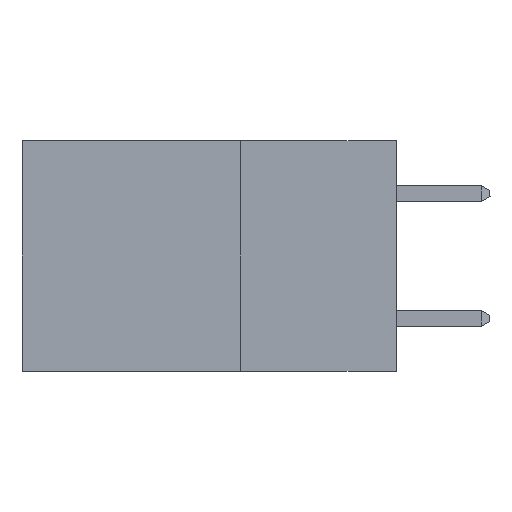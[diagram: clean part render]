
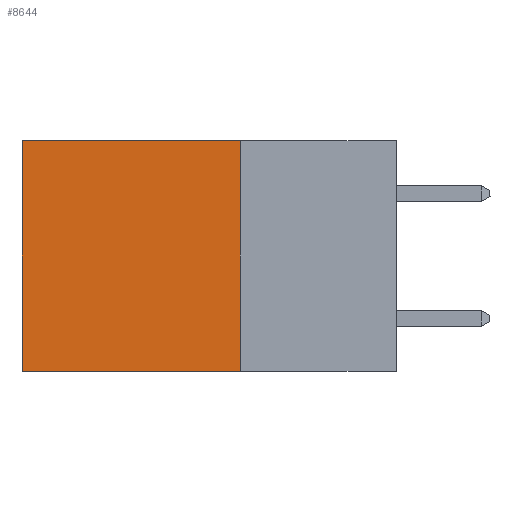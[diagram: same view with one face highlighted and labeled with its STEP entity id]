
A CAD part, left-side view. The second image highlights one B-rep face of the part: STEP entity #8644.
In plain terms, the highlighted planar face has unit normal (-1, 0, 0).
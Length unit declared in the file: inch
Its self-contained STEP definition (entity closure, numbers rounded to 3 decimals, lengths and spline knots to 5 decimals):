
#35 = VECTOR ( 'NONE', #12548, 39.37008 ) ;
#37 = AXIS2_PLACEMENT_3D ( 'NONE', #1441, #10226, #12680 ) ;
#749 = CARTESIAN_POINT ( 'NONE',  ( 0.298, 0.25, 0. ) ) ;
#1441 = CARTESIAN_POINT ( 'NONE',  ( 0.298, 0.25, 0. ) ) ;
#2020 = CARTESIAN_POINT ( 'NONE',  ( 0.298, 0.25, 0. ) ) ;
#2573 = ORIENTED_EDGE ( 'NONE', *, *, #11608, .T. ) ;
#3134 = LINE ( 'NONE', #9184, #35 ) ;
#3535 = EDGE_CURVE ( 'NONE', #3935, #13254, #6602, .T. ) ;
#3663 = DIRECTION ( 'NONE',  ( 0., 0., -1. ) ) ;
#3904 = VERTEX_POINT ( 'NONE', #749 ) ;
#3935 = VERTEX_POINT ( 'NONE', #10319 ) ;
#4289 = LINE ( 'NONE', #2020, #9448 ) ;
#5802 = CARTESIAN_POINT ( 'NONE',  ( 0.298, 0.25, -0.37 ) ) ;
#6526 = EDGE_CURVE ( 'NONE', #7617, #13254, #8835, .T. ) ;
#6602 = LINE ( 'NONE', #11719, #9190 ) ;
#6907 = ORIENTED_EDGE ( 'NONE', *, *, #9926, .F. ) ;
#7183 = ORIENTED_EDGE ( 'NONE', *, *, #6526, .F. ) ;
#7617 = VERTEX_POINT ( 'NONE', #5802 ) ;
#8644 = ADVANCED_FACE ( 'NONE', ( #12233 ), #11887, .F. ) ;
#8835 = LINE ( 'NONE', #12252, #14677 ) ;
#9184 = CARTESIAN_POINT ( 'NONE',  ( 0.298, 0.25, 0. ) ) ;
#9190 = VECTOR ( 'NONE', #3663, 39.37008 ) ;
#9373 = DIRECTION ( 'NONE',  ( 0., 0., -1. ) ) ;
#9448 = VECTOR ( 'NONE', #9373, 39.37008 ) ;
#9926 = EDGE_CURVE ( 'NONE', #3904, #7617, #4289, .T. ) ;
#10226 = DIRECTION ( 'NONE',  ( 1., 0., 0. ) ) ;
#10319 = CARTESIAN_POINT ( 'NONE',  ( 0.298, 0.6, 0. ) ) ;
#11464 = EDGE_LOOP ( 'NONE', ( #13954, #7183, #6907, #2573 ) ) ;
#11608 = EDGE_CURVE ( 'NONE', #3904, #3935, #3134, .T. ) ;
#11719 = CARTESIAN_POINT ( 'NONE',  ( 0.298, 0.6, 0. ) ) ;
#11887 = PLANE ( 'NONE',  #37 ) ;
#12233 = FACE_OUTER_BOUND ( 'NONE', #11464, .T. ) ;
#12252 = CARTESIAN_POINT ( 'NONE',  ( 0.298, 0.25, -0.37 ) ) ;
#12303 = DIRECTION ( 'NONE',  ( 0., 1., 0. ) ) ;
#12548 = DIRECTION ( 'NONE',  ( 0., 1., 0. ) ) ;
#12680 = DIRECTION ( 'NONE',  ( 0., 0., -1. ) ) ;
#13254 = VERTEX_POINT ( 'NONE', #14565 ) ;
#13954 = ORIENTED_EDGE ( 'NONE', *, *, #3535, .T. ) ;
#14565 = CARTESIAN_POINT ( 'NONE',  ( 0.298, 0.6, -0.37 ) ) ;
#14677 = VECTOR ( 'NONE', #12303, 39.37008 ) ;
